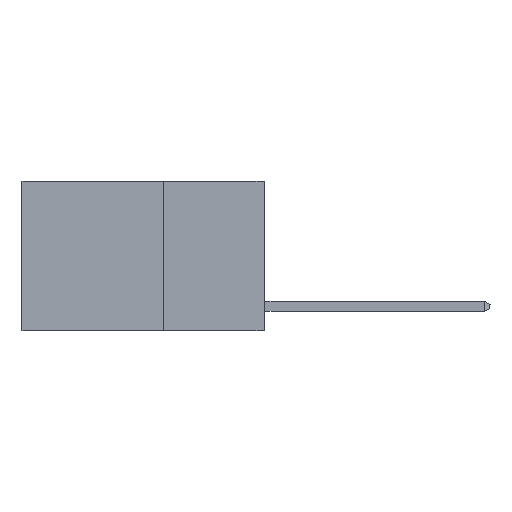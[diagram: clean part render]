
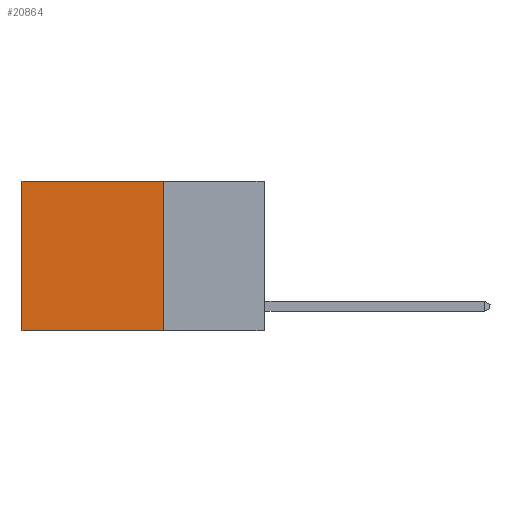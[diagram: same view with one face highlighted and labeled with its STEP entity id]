
A CAD part, left-side view. The second image highlights one B-rep face of the part: STEP entity #20864.
In plain terms, the highlighted planar face has unit normal (-1, 0, 0).
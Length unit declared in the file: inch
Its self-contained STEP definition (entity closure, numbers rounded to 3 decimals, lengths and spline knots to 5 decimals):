
#545 = VECTOR ( 'NONE', #3514, 39.37008 ) ;
#559 = EDGE_LOOP ( 'NONE', ( #17877, #15419, #13636, #15216 ) ) ;
#1374 = DIRECTION ( 'NONE',  ( 0., 0., -1. ) ) ;
#2291 = LINE ( 'NONE', #11334, #6958 ) ;
#3514 = DIRECTION ( 'NONE',  ( 0., 0., -1. ) ) ;
#3834 = PLANE ( 'NONE',  #9514 ) ;
#3951 = CARTESIAN_POINT ( 'NONE',  ( 0.2625, 0.25, 0. ) ) ;
#4209 = LINE ( 'NONE', #14683, #12959 ) ;
#4761 = DIRECTION ( 'NONE',  ( 0., 1., 0. ) ) ;
#5293 = CARTESIAN_POINT ( 'NONE',  ( 0.2625, 0.25, 0. ) ) ;
#5510 = CARTESIAN_POINT ( 'NONE',  ( 0.2625, 0.6, 0. ) ) ;
#5833 = DIRECTION ( 'NONE',  ( 0., 0., -1. ) ) ;
#6522 = EDGE_CURVE ( 'NONE', #20238, #24199, #12846, .T. ) ;
#6958 = VECTOR ( 'NONE', #1374, 39.37008 ) ;
#7323 = CARTESIAN_POINT ( 'NONE',  ( 0.2625, 0.25, -0.37 ) ) ;
#7630 = CARTESIAN_POINT ( 'NONE',  ( 0.2625, 0.6, -0.37 ) ) ;
#7755 = VERTEX_POINT ( 'NONE', #7323 ) ;
#9514 = AXIS2_PLACEMENT_3D ( 'NONE', #19655, #17736, #5833 ) ;
#10890 = EDGE_CURVE ( 'NONE', #7755, #23433, #4209, .T. ) ;
#11334 = CARTESIAN_POINT ( 'NONE',  ( 0.2625, 0.25, 0. ) ) ;
#12846 = LINE ( 'NONE', #5293, #21488 ) ;
#12959 = VECTOR ( 'NONE', #4761, 39.37008 ) ;
#13636 = ORIENTED_EDGE ( 'NONE', *, *, #15580, .F. ) ;
#13911 = EDGE_CURVE ( 'NONE', #24199, #23433, #22225, .T. ) ;
#14683 = CARTESIAN_POINT ( 'NONE',  ( 0.2625, 0.25, -0.37 ) ) ;
#15216 = ORIENTED_EDGE ( 'NONE', *, *, #6522, .T. ) ;
#15419 = ORIENTED_EDGE ( 'NONE', *, *, #10890, .F. ) ;
#15580 = EDGE_CURVE ( 'NONE', #20238, #7755, #2291, .T. ) ;
#17736 = DIRECTION ( 'NONE',  ( 1., 0., 0. ) ) ;
#17877 = ORIENTED_EDGE ( 'NONE', *, *, #13911, .T. ) ;
#19196 = DIRECTION ( 'NONE',  ( 0., 1., 0. ) ) ;
#19655 = CARTESIAN_POINT ( 'NONE',  ( 0.2625, 0.25, 0. ) ) ;
#20238 = VERTEX_POINT ( 'NONE', #3951 ) ;
#20864 = ADVANCED_FACE ( 'NONE', ( #21093 ), #3834, .F. ) ;
#21093 = FACE_OUTER_BOUND ( 'NONE', #559, .T. ) ;
#21488 = VECTOR ( 'NONE', #19196, 39.37008 ) ;
#21858 = CARTESIAN_POINT ( 'NONE',  ( 0.2625, 0.6, 0. ) ) ;
#22225 = LINE ( 'NONE', #5510, #545 ) ;
#23433 = VERTEX_POINT ( 'NONE', #7630 ) ;
#24199 = VERTEX_POINT ( 'NONE', #21858 ) ;
